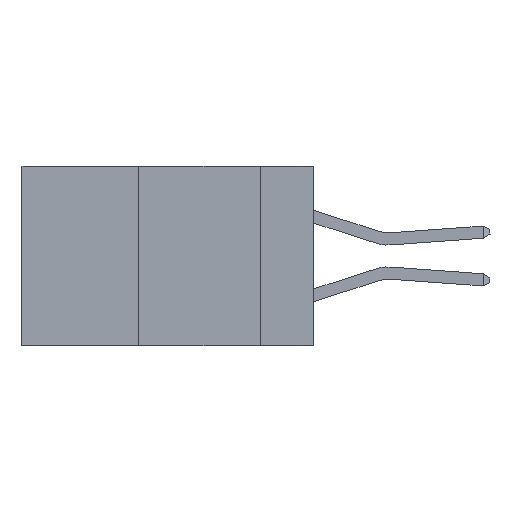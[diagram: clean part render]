
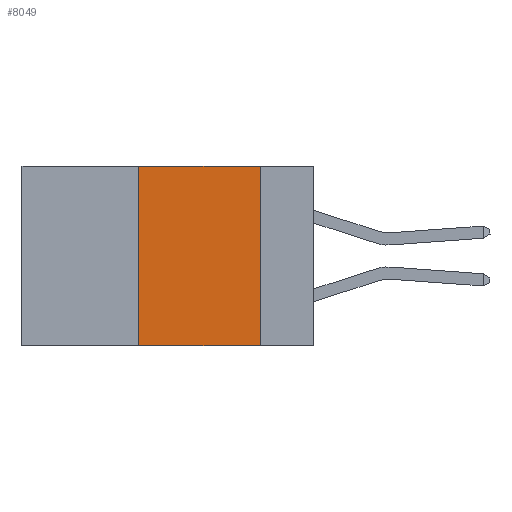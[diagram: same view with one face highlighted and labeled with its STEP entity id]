
A CAD part, left-side view. The second image highlights one B-rep face of the part: STEP entity #8049.
In plain terms, the highlighted planar face has unit normal (-1, 0, 0).
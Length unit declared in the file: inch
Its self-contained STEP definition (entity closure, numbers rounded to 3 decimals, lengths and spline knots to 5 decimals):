
#1900 = LINE ( 'NONE', #19310, #7723 ) ;
#3488 = VERTEX_POINT ( 'NONE', #13680 ) ;
#6119 = VERTEX_POINT ( 'NONE', #16925 ) ;
#6657 = ORIENTED_EDGE ( 'NONE', *, *, #19305, .F. ) ;
#7246 = VERTEX_POINT ( 'NONE', #13638 ) ;
#7723 = VECTOR ( 'NONE', #12951, 39.37008 ) ;
#8049 = ADVANCED_FACE ( 'NONE', ( #20448 ), #17302, .F. ) ;
#9828 = EDGE_LOOP ( 'NONE', ( #19539, #6657, #15419, #12337 ) ) ;
#10455 = LINE ( 'NONE', #15350, #10755 ) ;
#10649 = DIRECTION ( 'NONE',  ( 1., 0., 0. ) ) ;
#10755 = VECTOR ( 'NONE', #16913, 39.37008 ) ;
#11110 = EDGE_CURVE ( 'NONE', #3488, #7246, #1900, .T. ) ;
#12224 = CARTESIAN_POINT ( 'NONE',  ( 0., 0.6, 0. ) ) ;
#12337 = ORIENTED_EDGE ( 'NONE', *, *, #19150, .T. ) ;
#12566 = VECTOR ( 'NONE', #18604, 39.37008 ) ;
#12616 = EDGE_CURVE ( 'NONE', #15260, #6119, #10455, .T. ) ;
#12951 = DIRECTION ( 'NONE',  ( 0., 0., 1. ) ) ;
#13204 = CARTESIAN_POINT ( 'NONE',  ( 0., 0.11, 0. ) ) ;
#13384 = CARTESIAN_POINT ( 'NONE',  ( 0., 0.6, -0.37 ) ) ;
#13638 = CARTESIAN_POINT ( 'NONE',  ( 0., 0.36, 0. ) ) ;
#13680 = CARTESIAN_POINT ( 'NONE',  ( 0., 0.36, -0.37 ) ) ;
#14758 = LINE ( 'NONE', #13384, #15895 ) ;
#15260 = VERTEX_POINT ( 'NONE', #13204 ) ;
#15350 = CARTESIAN_POINT ( 'NONE',  ( 0., 0.11, 0. ) ) ;
#15377 = CARTESIAN_POINT ( 'NONE',  ( 0., 0.6, 0. ) ) ;
#15419 = ORIENTED_EDGE ( 'NONE', *, *, #11110, .F. ) ;
#15579 = LINE ( 'NONE', #15377, #12566 ) ;
#15895 = VECTOR ( 'NONE', #19660, 39.37008 ) ;
#16913 = DIRECTION ( 'NONE',  ( 0., 0., -1. ) ) ;
#16925 = CARTESIAN_POINT ( 'NONE',  ( 0., 0.11, -0.37 ) ) ;
#17302 = PLANE ( 'NONE',  #17725 ) ;
#17725 = AXIS2_PLACEMENT_3D ( 'NONE', #12224, #10649, #18871 ) ;
#18604 = DIRECTION ( 'NONE',  ( 0., -1., 0. ) ) ;
#18871 = DIRECTION ( 'NONE',  ( 0., 0., -1. ) ) ;
#19150 = EDGE_CURVE ( 'NONE', #3488, #6119, #14758, .T. ) ;
#19305 = EDGE_CURVE ( 'NONE', #7246, #15260, #15579, .T. ) ;
#19310 = CARTESIAN_POINT ( 'NONE',  ( 0., 0.36, 0. ) ) ;
#19539 = ORIENTED_EDGE ( 'NONE', *, *, #12616, .F. ) ;
#19660 = DIRECTION ( 'NONE',  ( 0., -1., 0. ) ) ;
#20448 = FACE_OUTER_BOUND ( 'NONE', #9828, .T. ) ;
